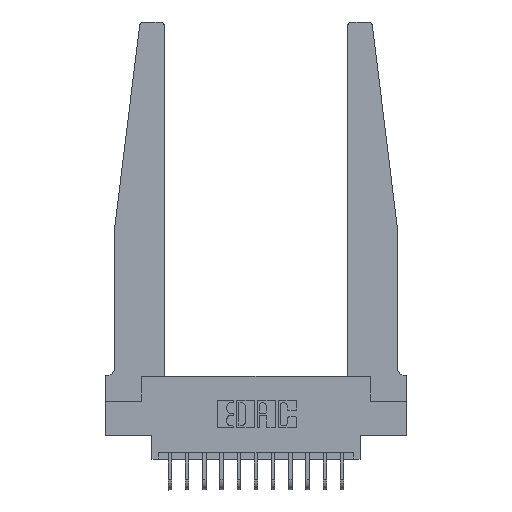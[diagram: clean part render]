
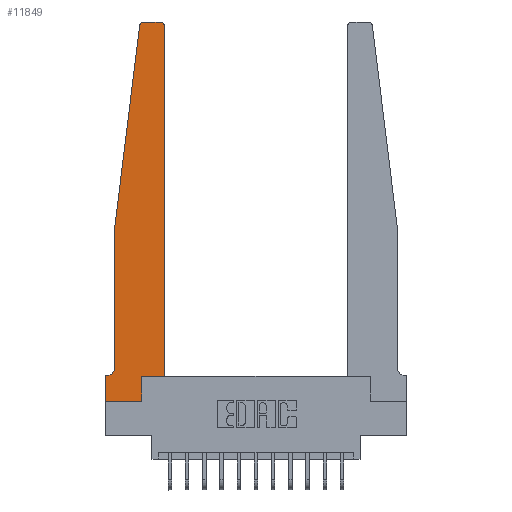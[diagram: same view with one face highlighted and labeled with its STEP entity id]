
A CAD part, top view. The second image highlights one B-rep face of the part: STEP entity #11849.
In plain terms, the highlighted planar face has unit normal (0, 0, 1).
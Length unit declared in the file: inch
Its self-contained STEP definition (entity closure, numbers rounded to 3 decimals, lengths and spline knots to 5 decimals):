
#60 = AXIS2_PLACEMENT_3D ( 'NONE', #1591, #11311, #4378 ) ;
#99 = VERTEX_POINT ( 'NONE', #9045 ) ;
#119 = VERTEX_POINT ( 'NONE', #9204 ) ;
#405 = DIRECTION ( 'NONE',  ( 0., 0., 1. ) ) ;
#526 = AXIS2_PLACEMENT_3D ( 'NONE', #5898, #405, #14192 ) ;
#589 = EDGE_CURVE ( 'NONE', #119, #4636, #13590, .T. ) ;
#597 = DIRECTION ( 'NONE',  ( 1., 0., 0. ) ) ;
#848 = LINE ( 'NONE', #8819, #1918 ) ;
#866 = CARTESIAN_POINT ( 'NONE',  ( 0.395, 2.75, 0.37 ) ) ;
#871 = FACE_OUTER_BOUND ( 'NONE', #14084, .T. ) ;
#952 = LINE ( 'NONE', #11303, #11396 ) ;
#954 = DIRECTION ( 'NONE',  ( -1., 0., 0. ) ) ;
#1102 = VECTOR ( 'NONE', #10522, 39.37008 ) ;
#1404 = VECTOR ( 'NONE', #14304, 39.37008 ) ;
#1484 = CARTESIAN_POINT ( 'NONE',  ( 0.425, 0.18, 0.37 ) ) ;
#1591 = CARTESIAN_POINT ( 'NONE',  ( 0., 0.1875, 0.37 ) ) ;
#1628 = DIRECTION ( 'NONE',  ( -0.122, -0.992, 0. ) ) ;
#1815 = EDGE_CURVE ( 'NONE', #13471, #99, #952, .T. ) ;
#1859 = AXIS2_PLACEMENT_3D ( 'NONE', #11165, #2638, #2838 ) ;
#1918 = VECTOR ( 'NONE', #10198, 39.37008 ) ;
#1973 = DIRECTION ( 'NONE',  ( 1., 0., 0. ) ) ;
#2051 = CARTESIAN_POINT ( 'NONE',  ( 0.27653, 2.75, 0.37 ) ) ;
#2260 = DIRECTION ( 'NONE',  ( 0., -1., 0. ) ) ;
#2439 = VECTOR ( 'NONE', #597, 39.37008 ) ;
#2638 = DIRECTION ( 'NONE',  ( 0., 0., 1. ) ) ;
#2728 = VERTEX_POINT ( 'NONE', #866 ) ;
#2828 = ORIENTED_EDGE ( 'NONE', *, *, #4319, .T. ) ;
#2838 = DIRECTION ( 'NONE',  ( 1., 0., 0. ) ) ;
#2926 = LINE ( 'NONE', #10371, #7294 ) ;
#3525 = CARTESIAN_POINT ( 'NONE',  ( 0.425, 0.18, 0.37 ) ) ;
#3596 = EDGE_CURVE ( 'NONE', #4636, #13471, #6575, .T. ) ;
#3704 = CIRCLE ( 'NONE', #1859, 0.03 ) ;
#4135 = CARTESIAN_POINT ( 'NONE',  ( 0., 0., 0.37 ) ) ;
#4263 = EDGE_CURVE ( 'NONE', #16818, #8790, #15898, .T. ) ;
#4302 = ORIENTED_EDGE ( 'NONE', *, *, #3596, .T. ) ;
#4319 = EDGE_CURVE ( 'NONE', #11487, #5464, #3704, .T. ) ;
#4378 = DIRECTION ( 'NONE',  ( 1., 0., 0. ) ) ;
#4636 = VERTEX_POINT ( 'NONE', #4135 ) ;
#4668 = CARTESIAN_POINT ( 'NONE',  ( 0.425, 0.18, 0.37 ) ) ;
#4750 = CARTESIAN_POINT ( 'NONE',  ( 0., 0., 0.37 ) ) ;
#4953 = ORIENTED_EDGE ( 'NONE', *, *, #8892, .T. ) ;
#5464 = VERTEX_POINT ( 'NONE', #14148 ) ;
#5898 = CARTESIAN_POINT ( 'NONE',  ( 0.395, 2.72, 0.37 ) ) ;
#6134 = CARTESIAN_POINT ( 'NONE',  ( 0.2605, 0., 0.37 ) ) ;
#6395 = VERTEX_POINT ( 'NONE', #16464 ) ;
#6575 = LINE ( 'NONE', #8404, #16808 ) ;
#6651 = DIRECTION ( 'NONE',  ( 0., -1., 0. ) ) ;
#6763 = CARTESIAN_POINT ( 'NONE',  ( 0.425, 2.72, 0.37 ) ) ;
#6902 = ORIENTED_EDGE ( 'NONE', *, *, #17254, .T. ) ;
#7294 = VECTOR ( 'NONE', #2260, 39.37008 ) ;
#7830 = CIRCLE ( 'NONE', #526, 0.03 ) ;
#7862 = ORIENTED_EDGE ( 'NONE', *, *, #16552, .T. ) ;
#7951 = CARTESIAN_POINT ( 'NONE',  ( 0.015, 0.2375, 0.37 ) ) ;
#8193 = ORIENTED_EDGE ( 'NONE', *, *, #10891, .T. ) ;
#8326 = ORIENTED_EDGE ( 'NONE', *, *, #13710, .T. ) ;
#8371 = CARTESIAN_POINT ( 'NONE',  ( 0.065, 1.25, 0.37 ) ) ;
#8404 = CARTESIAN_POINT ( 'NONE',  ( 0., 0., 0.37 ) ) ;
#8523 = PLANE ( 'NONE',  #60 ) ;
#8527 = EDGE_CURVE ( 'NONE', #5464, #17491, #10110, .T. ) ;
#8566 = ORIENTED_EDGE ( 'NONE', *, *, #589, .T. ) ;
#8612 = EDGE_CURVE ( 'NONE', #6395, #119, #13346, .T. ) ;
#8639 = DIRECTION ( 'NONE',  ( 0., 1., 0. ) ) ;
#8790 = VERTEX_POINT ( 'NONE', #6763 ) ;
#8819 = CARTESIAN_POINT ( 'NONE',  ( 0.25, 2.75, 0.37 ) ) ;
#8892 = EDGE_CURVE ( 'NONE', #17491, #10863, #2926, .T. ) ;
#8993 = LINE ( 'NONE', #4668, #2439 ) ;
#9045 = CARTESIAN_POINT ( 'NONE',  ( 0.2605, 0.18, 0.37 ) ) ;
#9204 = CARTESIAN_POINT ( 'NONE',  ( 0., 0.1875, 0.37 ) ) ;
#10110 = LINE ( 'NONE', #15635, #12936 ) ;
#10198 = DIRECTION ( 'NONE',  ( -1., 0., 0. ) ) ;
#10371 = CARTESIAN_POINT ( 'NONE',  ( 0.065, 1.25, 0.37 ) ) ;
#10522 = DIRECTION ( 'NONE',  ( 0., 1., 0. ) ) ;
#10826 = ORIENTED_EDGE ( 'NONE', *, *, #1815, .T. ) ;
#10863 = VERTEX_POINT ( 'NONE', #13884 ) ;
#10891 = EDGE_CURVE ( 'NONE', #8790, #2728, #7830, .T. ) ;
#11165 = CARTESIAN_POINT ( 'NONE',  ( 0.27653, 2.72, 0.37 ) ) ;
#11303 = CARTESIAN_POINT ( 'NONE',  ( 0.2605, 0.18, 0.37 ) ) ;
#11311 = DIRECTION ( 'NONE',  ( 0., 0., 1. ) ) ;
#11396 = VECTOR ( 'NONE', #8639, 39.37008 ) ;
#11400 = CIRCLE ( 'NONE', #17616, 0.05 ) ;
#11487 = VERTEX_POINT ( 'NONE', #2051 ) ;
#11849 = ADVANCED_FACE ( 'NONE', ( #871 ), #8523, .T. ) ;
#12936 = VECTOR ( 'NONE', #1628, 39.37008 ) ;
#13346 = LINE ( 'NONE', #15826, #1404 ) ;
#13471 = VERTEX_POINT ( 'NONE', #6134 ) ;
#13513 = DIRECTION ( 'NONE',  ( 0., 0., -1. ) ) ;
#13590 = LINE ( 'NONE', #4750, #14234 ) ;
#13710 = EDGE_CURVE ( 'NONE', #2728, #11487, #848, .T. ) ;
#13884 = CARTESIAN_POINT ( 'NONE',  ( 0.065, 0.2375, 0.37 ) ) ;
#14084 = EDGE_LOOP ( 'NONE', ( #8326, #2828, #16595, #4953, #7862, #15852, #8566, #4302, #10826, #6902, #16165, #8193 ) ) ;
#14148 = CARTESIAN_POINT ( 'NONE',  ( 0.24675, 2.72367, 0.37 ) ) ;
#14192 = DIRECTION ( 'NONE',  ( 1., 0., 0. ) ) ;
#14234 = VECTOR ( 'NONE', #6651, 39.37008 ) ;
#14304 = DIRECTION ( 'NONE',  ( -1., 0., 0. ) ) ;
#15635 = CARTESIAN_POINT ( 'NONE',  ( 0.065, 1.25, 0.37 ) ) ;
#15826 = CARTESIAN_POINT ( 'NONE',  ( 0.065, 0.1875, 0.37 ) ) ;
#15852 = ORIENTED_EDGE ( 'NONE', *, *, #8612, .T. ) ;
#15898 = LINE ( 'NONE', #3525, #1102 ) ;
#16165 = ORIENTED_EDGE ( 'NONE', *, *, #4263, .T. ) ;
#16464 = CARTESIAN_POINT ( 'NONE',  ( 0.015, 0.1875, 0.37 ) ) ;
#16552 = EDGE_CURVE ( 'NONE', #10863, #6395, #11400, .T. ) ;
#16595 = ORIENTED_EDGE ( 'NONE', *, *, #8527, .T. ) ;
#16808 = VECTOR ( 'NONE', #1973, 39.37008 ) ;
#16818 = VERTEX_POINT ( 'NONE', #1484 ) ;
#17254 = EDGE_CURVE ( 'NONE', #99, #16818, #8993, .T. ) ;
#17491 = VERTEX_POINT ( 'NONE', #8371 ) ;
#17616 = AXIS2_PLACEMENT_3D ( 'NONE', #7951, #13513, #954 ) ;
